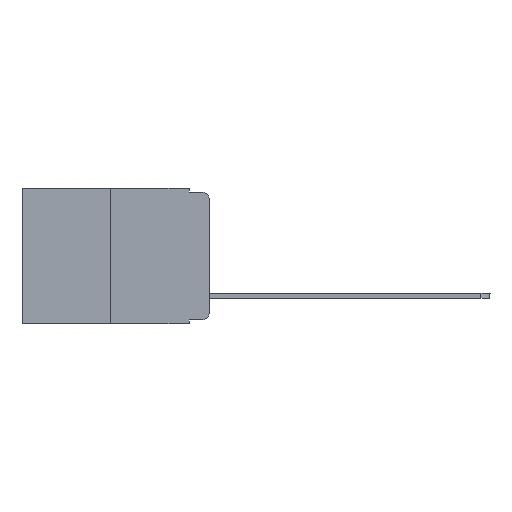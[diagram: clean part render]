
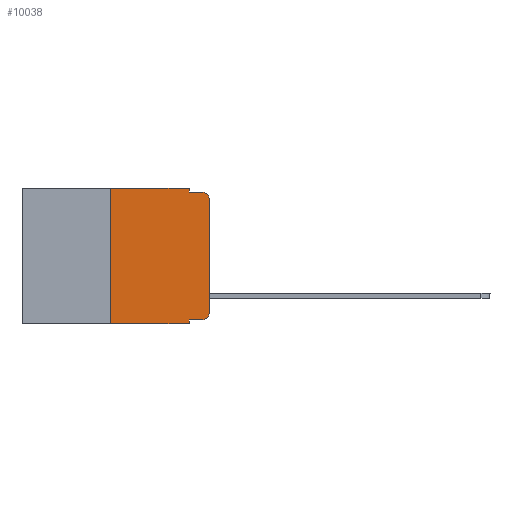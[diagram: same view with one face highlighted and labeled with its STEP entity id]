
A CAD part, left-side view. The second image highlights one B-rep face of the part: STEP entity #10038.
In plain terms, the highlighted planar face has unit normal (-1, 0, 0).
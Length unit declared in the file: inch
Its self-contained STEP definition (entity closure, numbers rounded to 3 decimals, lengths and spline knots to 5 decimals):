
#76 = DIRECTION ( 'NONE',  ( 0., 0., 1. ) ) ;
#302 = AXIS2_PLACEMENT_3D ( 'NONE', #12941, #2796, #2716 ) ;
#404 = EDGE_CURVE ( 'NONE', #1720, #11558, #15569, .T. ) ;
#583 = ORIENTED_EDGE ( 'NONE', *, *, #1128, .T. ) ;
#877 = VECTOR ( 'NONE', #16062, 39.37008 ) ;
#942 = ORIENTED_EDGE ( 'NONE', *, *, #5132, .T. ) ;
#992 = CARTESIAN_POINT ( 'NONE',  ( 0., 0.051, -0.343 ) ) ;
#1008 = VECTOR ( 'NONE', #3350, 39.37008 ) ;
#1058 = DIRECTION ( 'NONE',  ( 0., 0., -1. ) ) ;
#1065 = EDGE_CURVE ( 'NONE', #11558, #5894, #10992, .T. ) ;
#1066 = ORIENTED_EDGE ( 'NONE', *, *, #404, .F. ) ;
#1128 = EDGE_CURVE ( 'NONE', #11781, #14054, #4447, .T. ) ;
#1301 = VECTOR ( 'NONE', #13490, 39.37008 ) ;
#1369 = CARTESIAN_POINT ( 'NONE',  ( 0., 0.473, -0.343 ) ) ;
#1673 = LINE ( 'NONE', #6633, #8552 ) ;
#1720 = VERTEX_POINT ( 'NONE', #4363 ) ;
#1766 = DIRECTION ( 'NONE',  ( 0., 0., -1. ) ) ;
#2133 = ORIENTED_EDGE ( 'NONE', *, *, #3373, .T. ) ;
#2142 = CARTESIAN_POINT ( 'NONE',  ( 0., 0.25, -0.343 ) ) ;
#2224 = VECTOR ( 'NONE', #4650, 39.37008 ) ;
#2711 = CARTESIAN_POINT ( 'NONE',  ( 0., 0.02, -0.03 ) ) ;
#2716 = DIRECTION ( 'NONE',  ( 0., 0., -1. ) ) ;
#2796 = DIRECTION ( 'NONE',  ( -1., 0., 0. ) ) ;
#3091 = VECTOR ( 'NONE', #76, 39.37008 ) ;
#3350 = DIRECTION ( 'NONE',  ( 0., -1., 0. ) ) ;
#3373 = EDGE_CURVE ( 'NONE', #13662, #5894, #10021, .T. ) ;
#4020 = EDGE_CURVE ( 'NONE', #4956, #1720, #9636, .T. ) ;
#4338 = VERTEX_POINT ( 'NONE', #992 ) ;
#4361 = ORIENTED_EDGE ( 'NONE', *, *, #1065, .F. ) ;
#4363 = CARTESIAN_POINT ( 'NONE',  ( 0., 0.051, 0. ) ) ;
#4447 = CIRCLE ( 'NONE', #302, 0.02 ) ;
#4650 = DIRECTION ( 'NONE',  ( 0., 0., 1. ) ) ;
#4733 = CARTESIAN_POINT ( 'NONE',  ( 0., 0., 0. ) ) ;
#4956 = VERTEX_POINT ( 'NONE', #9380 ) ;
#4976 = LINE ( 'NONE', #8678, #1008 ) ;
#5132 = EDGE_CURVE ( 'NONE', #13612, #4338, #6239, .T. ) ;
#5675 = ORIENTED_EDGE ( 'NONE', *, *, #7613, .F. ) ;
#5834 = FACE_OUTER_BOUND ( 'NONE', #15332, .T. ) ;
#5894 = VERTEX_POINT ( 'NONE', #9955 ) ;
#6239 = LINE ( 'NONE', #1369, #7760 ) ;
#6245 = CARTESIAN_POINT ( 'NONE',  ( 0., 0.051, -0.333 ) ) ;
#6327 = LINE ( 'NONE', #7660, #3091 ) ;
#6633 = CARTESIAN_POINT ( 'NONE',  ( 0., 0.051, 0. ) ) ;
#7409 = CARTESIAN_POINT ( 'NONE',  ( 0., 0., -0.313 ) ) ;
#7462 = CARTESIAN_POINT ( 'NONE',  ( 0., 0.02, -0.333 ) ) ;
#7613 = EDGE_CURVE ( 'NONE', #13612, #4956, #6327, .T. ) ;
#7660 = CARTESIAN_POINT ( 'NONE',  ( 0., 0.25, 0. ) ) ;
#7760 = VECTOR ( 'NONE', #13891, 39.37008 ) ;
#8258 = DIRECTION ( 'NONE',  ( 0., 0., -1. ) ) ;
#8324 = CARTESIAN_POINT ( 'NONE',  ( 0., 0.473, 0. ) ) ;
#8552 = VECTOR ( 'NONE', #8258, 39.37008 ) ;
#8678 = CARTESIAN_POINT ( 'NONE',  ( 0., 0.051, -0.333 ) ) ;
#9202 = VECTOR ( 'NONE', #1766, 39.37008 ) ;
#9305 = ORIENTED_EDGE ( 'NONE', *, *, #15319, .T. ) ;
#9380 = CARTESIAN_POINT ( 'NONE',  ( 0., 0.25, 0. ) ) ;
#9636 = LINE ( 'NONE', #8324, #1301 ) ;
#9765 = CARTESIAN_POINT ( 'NONE',  ( 0., 0.051, -0.01 ) ) ;
#9955 = CARTESIAN_POINT ( 'NONE',  ( 0., 0.02, -0.01 ) ) ;
#10021 = CIRCLE ( 'NONE', #13959, 0.02 ) ;
#10038 = ADVANCED_FACE ( 'NONE', ( #5834 ), #10845, .F. ) ;
#10385 = ORIENTED_EDGE ( 'NONE', *, *, #13501, .F. ) ;
#10845 = PLANE ( 'NONE',  #16081 ) ;
#10968 = CARTESIAN_POINT ( 'NONE',  ( 0., 0., -0.03 ) ) ;
#10992 = LINE ( 'NONE', #12383, #877 ) ;
#11355 = VERTEX_POINT ( 'NONE', #6245 ) ;
#11558 = VERTEX_POINT ( 'NONE', #9765 ) ;
#11660 = CARTESIAN_POINT ( 'NONE',  ( 0., 0.051, 0. ) ) ;
#11781 = VERTEX_POINT ( 'NONE', #7462 ) ;
#11941 = ORIENTED_EDGE ( 'NONE', *, *, #4020, .F. ) ;
#12116 = LINE ( 'NONE', #4733, #2224 ) ;
#12250 = DIRECTION ( 'NONE',  ( 1., 0., 0. ) ) ;
#12383 = CARTESIAN_POINT ( 'NONE',  ( 0., 0.051, -0.01 ) ) ;
#12548 = DIRECTION ( 'NONE',  ( -1., 0., 0. ) ) ;
#12941 = CARTESIAN_POINT ( 'NONE',  ( 0., 0.02, -0.313 ) ) ;
#13475 = CARTESIAN_POINT ( 'NONE',  ( 0., 0.473, 0. ) ) ;
#13490 = DIRECTION ( 'NONE',  ( 0., -1., 0. ) ) ;
#13501 = EDGE_CURVE ( 'NONE', #11355, #4338, #1673, .T. ) ;
#13579 = EDGE_CURVE ( 'NONE', #11355, #11781, #4976, .T. ) ;
#13612 = VERTEX_POINT ( 'NONE', #2142 ) ;
#13662 = VERTEX_POINT ( 'NONE', #10968 ) ;
#13776 = DIRECTION ( 'NONE',  ( 0., 0., -1. ) ) ;
#13891 = DIRECTION ( 'NONE',  ( 0., -1., 0. ) ) ;
#13959 = AXIS2_PLACEMENT_3D ( 'NONE', #2711, #12548, #13776 ) ;
#14054 = VERTEX_POINT ( 'NONE', #7409 ) ;
#15319 = EDGE_CURVE ( 'NONE', #14054, #13662, #12116, .T. ) ;
#15332 = EDGE_LOOP ( 'NONE', ( #9305, #2133, #4361, #1066, #11941, #5675, #942, #10385, #15776, #583 ) ) ;
#15569 = LINE ( 'NONE', #11660, #9202 ) ;
#15776 = ORIENTED_EDGE ( 'NONE', *, *, #13579, .T. ) ;
#16062 = DIRECTION ( 'NONE',  ( 0., -1., 0. ) ) ;
#16081 = AXIS2_PLACEMENT_3D ( 'NONE', #13475, #12250, #1058 ) ;
